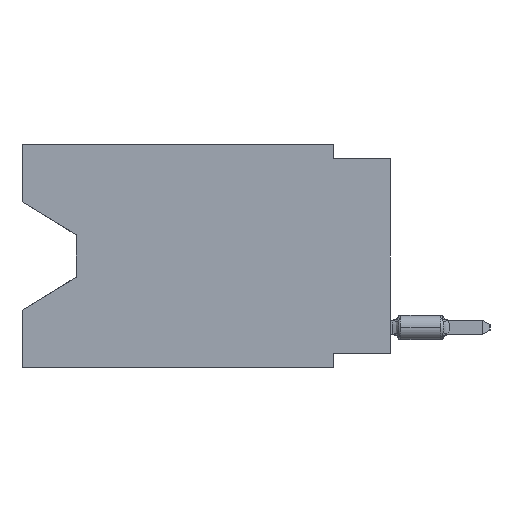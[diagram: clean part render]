
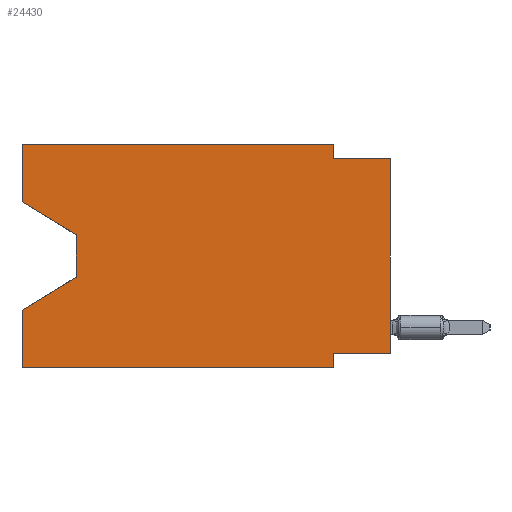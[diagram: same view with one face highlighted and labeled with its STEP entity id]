
A CAD part, left-side view. The second image highlights one B-rep face of the part: STEP entity #24430.
In plain terms, the highlighted planar face has unit normal (-1, 0, 0).
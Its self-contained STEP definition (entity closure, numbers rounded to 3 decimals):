
#602 = ORIENTED_EDGE ( 'NONE', *, *, #11021, .F. ) ;
#1420 = EDGE_CURVE ( 'NONE', #1979, #18576, #2364, .T. ) ;
#1866 = VERTEX_POINT ( 'NONE', #15323 ) ;
#1905 = EDGE_CURVE ( 'NONE', #27083, #25141, #24600, .T. ) ;
#1979 = VERTEX_POINT ( 'NONE', #24089 ) ;
#2130 = DIRECTION ( 'NONE',  ( 0., 0., 1. ) ) ;
#2364 = LINE ( 'NONE', #34145, #20522 ) ;
#2519 = ORIENTED_EDGE ( 'NONE', *, *, #12651, .T. ) ;
#2623 = LINE ( 'NONE', #15978, #34398 ) ;
#3172 = DIRECTION ( 'NONE',  ( 0., 0., 1. ) ) ;
#3803 = VERTEX_POINT ( 'NONE', #32383 ) ;
#4130 = CARTESIAN_POINT ( 'NONE',  ( 0., 0., -0.635 ) ) ;
#4137 = ORIENTED_EDGE ( 'NONE', *, *, #4808, .F. ) ;
#4235 = CARTESIAN_POINT ( 'NONE',  ( 0., 16.383, -9.906 ) ) ;
#4808 = EDGE_CURVE ( 'NONE', #3803, #1979, #2623, .T. ) ;
#4944 = DIRECTION ( 'NONE',  ( 0., 0., -1. ) ) ;
#5267 = LINE ( 'NONE', #7554, #17026 ) ;
#5749 = DIRECTION ( 'NONE',  ( 0., 0., -1. ) ) ;
#6122 = VECTOR ( 'NONE', #19048, 1000. ) ;
#6482 = ORIENTED_EDGE ( 'NONE', *, *, #27572, .F. ) ;
#6655 = LINE ( 'NONE', #25626, #8955 ) ;
#7005 = ORIENTED_EDGE ( 'NONE', *, *, #1905, .T. ) ;
#7306 = VECTOR ( 'NONE', #5749, 1000. ) ;
#7369 = VERTEX_POINT ( 'NONE', #32204 ) ;
#7381 = CARTESIAN_POINT ( 'NONE',  ( 0., 2.54, -9.906 ) ) ;
#7554 = CARTESIAN_POINT ( 'NONE',  ( 0., 0., 0. ) ) ;
#7584 = CARTESIAN_POINT ( 'NONE',  ( 0., 13.97, -4.013 ) ) ;
#8041 = LINE ( 'NONE', #7381, #7306 ) ;
#8369 = DIRECTION ( 'NONE',  ( 0., 1., 0. ) ) ;
#8912 = AXIS2_PLACEMENT_3D ( 'NONE', #26218, #31491, #15165 ) ;
#8955 = VECTOR ( 'NONE', #20184, 1000. ) ;
#9420 = ORIENTED_EDGE ( 'NONE', *, *, #10614, .F. ) ;
#9821 = CARTESIAN_POINT ( 'NONE',  ( 0., 16.383, -7.36 ) ) ;
#10327 = VECTOR ( 'NONE', #4944, 1000. ) ;
#10614 = EDGE_CURVE ( 'NONE', #14880, #18795, #24369, .T. ) ;
#10995 = CARTESIAN_POINT ( 'NONE',  ( 0., 13.97, -4.013 ) ) ;
#11021 = EDGE_CURVE ( 'NONE', #1866, #3803, #16768, .T. ) ;
#11076 = DIRECTION ( 'NONE',  ( 0., 0.855, -0.519 ) ) ;
#12173 = CARTESIAN_POINT ( 'NONE',  ( 0., 16.383, -9.906 ) ) ;
#12651 = EDGE_CURVE ( 'NONE', #13044, #31915, #33773, .T. ) ;
#12801 = VECTOR ( 'NONE', #8369, 1000. ) ;
#13044 = VERTEX_POINT ( 'NONE', #4235 ) ;
#13076 = DIRECTION ( 'NONE',  ( 0., -1., 0. ) ) ;
#13522 = ORIENTED_EDGE ( 'NONE', *, *, #25132, .T. ) ;
#13726 = CARTESIAN_POINT ( 'NONE',  ( 0., 13.97, -5.893 ) ) ;
#13903 = EDGE_CURVE ( 'NONE', #14880, #18576, #5267, .T. ) ;
#14880 = VERTEX_POINT ( 'NONE', #29454 ) ;
#14922 = VERTEX_POINT ( 'NONE', #10995 ) ;
#15153 = DIRECTION ( 'NONE',  ( 0., -1., 0. ) ) ;
#15165 = DIRECTION ( 'NONE',  ( 0., 0., -1. ) ) ;
#15323 = CARTESIAN_POINT ( 'NONE',  ( 0., 16.383, 0. ) ) ;
#15978 = CARTESIAN_POINT ( 'NONE',  ( 0., 2.54, 0. ) ) ;
#16768 = LINE ( 'NONE', #26774, #6122 ) ;
#17026 = VECTOR ( 'NONE', #32130, 1000. ) ;
#18158 = FACE_OUTER_BOUND ( 'NONE', #27988, .T. ) ;
#18576 = VERTEX_POINT ( 'NONE', #4130 ) ;
#18795 = VERTEX_POINT ( 'NONE', #34658 ) ;
#18948 = DIRECTION ( 'NONE',  ( 0., 0., -1. ) ) ;
#19000 = ORIENTED_EDGE ( 'NONE', *, *, #13903, .T. ) ;
#19048 = DIRECTION ( 'NONE',  ( 0., -1., 0. ) ) ;
#19724 = LINE ( 'NONE', #7584, #10327 ) ;
#20184 = DIRECTION ( 'NONE',  ( 0., -0.855, -0.519 ) ) ;
#20522 = VECTOR ( 'NONE', #13076, 1000. ) ;
#20569 = CARTESIAN_POINT ( 'NONE',  ( 0., 16.383, 0. ) ) ;
#21680 = ORIENTED_EDGE ( 'NONE', *, *, #31768, .T. ) ;
#22897 = ORIENTED_EDGE ( 'NONE', *, *, #1420, .F. ) ;
#23047 = VECTOR ( 'NONE', #3172, 1000. ) ;
#23590 = VECTOR ( 'NONE', #15153, 1000. ) ;
#24089 = CARTESIAN_POINT ( 'NONE',  ( 0., 2.54, -0.635 ) ) ;
#24369 = LINE ( 'NONE', #26820, #12801 ) ;
#24430 = ADVANCED_FACE ( 'NONE', ( #18158 ), #34297, .F. ) ;
#24600 = LINE ( 'NONE', #13726, #25287 ) ;
#25132 = EDGE_CURVE ( 'NONE', #7369, #14922, #6655, .T. ) ;
#25141 = VERTEX_POINT ( 'NONE', #9821 ) ;
#25287 = VECTOR ( 'NONE', #11076, 1000. ) ;
#25506 = LINE ( 'NONE', #20569, #26925 ) ;
#25626 = CARTESIAN_POINT ( 'NONE',  ( 0., 16.383, -2.546 ) ) ;
#25889 = EDGE_CURVE ( 'NONE', #13044, #25141, #25506, .T. ) ;
#26218 = CARTESIAN_POINT ( 'NONE',  ( 0., 16.383, 0. ) ) ;
#26774 = CARTESIAN_POINT ( 'NONE',  ( 0., 16.383, 0. ) ) ;
#26820 = CARTESIAN_POINT ( 'NONE',  ( 0., 0., -9.271 ) ) ;
#26925 = VECTOR ( 'NONE', #2130, 1000. ) ;
#27083 = VERTEX_POINT ( 'NONE', #30487 ) ;
#27223 = CARTESIAN_POINT ( 'NONE',  ( 0., 16.383, 0. ) ) ;
#27572 = EDGE_CURVE ( 'NONE', #18795, #31915, #8041, .T. ) ;
#27750 = ORIENTED_EDGE ( 'NONE', *, *, #25889, .F. ) ;
#27820 = EDGE_CURVE ( 'NONE', #7369, #1866, #29857, .T. ) ;
#27988 = EDGE_LOOP ( 'NONE', ( #13522, #21680, #7005, #27750, #2519, #6482, #9420, #19000, #22897, #4137, #602, #30805 ) ) ;
#29454 = CARTESIAN_POINT ( 'NONE',  ( 0., 0., -9.271 ) ) ;
#29857 = LINE ( 'NONE', #27223, #23047 ) ;
#30487 = CARTESIAN_POINT ( 'NONE',  ( 0., 13.97, -5.893 ) ) ;
#30805 = ORIENTED_EDGE ( 'NONE', *, *, #27820, .F. ) ;
#31465 = CARTESIAN_POINT ( 'NONE',  ( 0., 2.54, -9.906 ) ) ;
#31491 = DIRECTION ( 'NONE',  ( 1., 0., 0. ) ) ;
#31768 = EDGE_CURVE ( 'NONE', #14922, #27083, #19724, .T. ) ;
#31915 = VERTEX_POINT ( 'NONE', #31465 ) ;
#32130 = DIRECTION ( 'NONE',  ( 0., 0., 1. ) ) ;
#32204 = CARTESIAN_POINT ( 'NONE',  ( 0., 16.383, -2.546 ) ) ;
#32383 = CARTESIAN_POINT ( 'NONE',  ( 0., 2.54, 0. ) ) ;
#33773 = LINE ( 'NONE', #12173, #23590 ) ;
#34145 = CARTESIAN_POINT ( 'NONE',  ( 0., 0., -0.635 ) ) ;
#34297 = PLANE ( 'NONE',  #8912 ) ;
#34398 = VECTOR ( 'NONE', #18948, 1000. ) ;
#34658 = CARTESIAN_POINT ( 'NONE',  ( 0., 2.54, -9.271 ) ) ;
